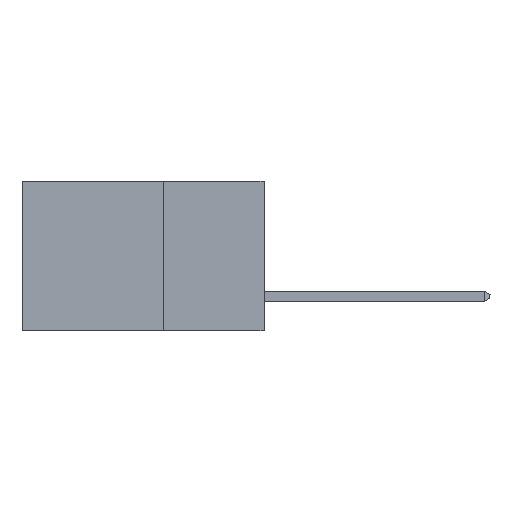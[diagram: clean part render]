
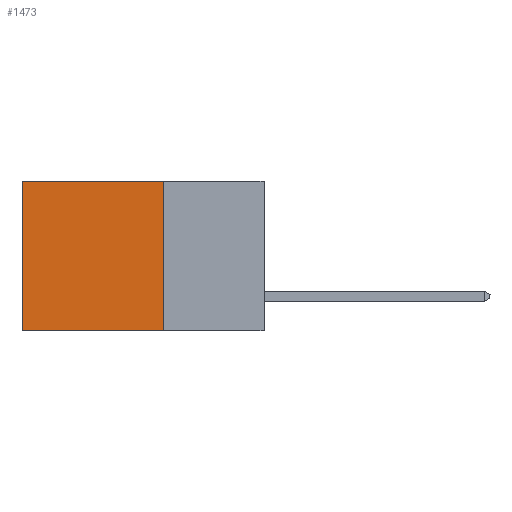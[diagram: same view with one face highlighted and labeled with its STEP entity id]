
A CAD part, left-side view. The second image highlights one B-rep face of the part: STEP entity #1473.
In plain terms, the highlighted planar face has unit normal (-1, 0, 0).
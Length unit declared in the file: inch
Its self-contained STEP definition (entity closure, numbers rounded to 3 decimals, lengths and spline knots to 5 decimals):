
#175 = CARTESIAN_POINT ( 'NONE',  ( 0.2615, 0.25, -0.37 ) ) ;
#930 = VECTOR ( 'NONE', #11636, 39.37008 ) ;
#1304 = EDGE_LOOP ( 'NONE', ( #3602, #11154, #7606, #9741 ) ) ;
#1473 = ADVANCED_FACE ( 'NONE', ( #2576 ), #13557, .F. ) ;
#1563 = DIRECTION ( 'NONE',  ( 0., 0., -1. ) ) ;
#2576 = FACE_OUTER_BOUND ( 'NONE', #1304, .T. ) ;
#3214 = CARTESIAN_POINT ( 'NONE',  ( 0.2615, 0.25, -0.37 ) ) ;
#3551 = CARTESIAN_POINT ( 'NONE',  ( 0.2615, 0.25, 0. ) ) ;
#3602 = ORIENTED_EDGE ( 'NONE', *, *, #7411, .T. ) ;
#3848 = LINE ( 'NONE', #4694, #7327 ) ;
#3891 = CARTESIAN_POINT ( 'NONE',  ( 0.2615, 0.6, -0.37 ) ) ;
#3955 = LINE ( 'NONE', #5013, #13419 ) ;
#4158 = DIRECTION ( 'NONE',  ( 1., 0., 0. ) ) ;
#4160 = EDGE_CURVE ( 'NONE', #10025, #10816, #3955, .T. ) ;
#4694 = CARTESIAN_POINT ( 'NONE',  ( 0.2615, 0.6, -0.37 ) ) ;
#5013 = CARTESIAN_POINT ( 'NONE',  ( 0.2615, 0.25, -0.37 ) ) ;
#5068 = VERTEX_POINT ( 'NONE', #3891 ) ;
#5295 = LINE ( 'NONE', #13931, #12448 ) ;
#6496 = DIRECTION ( 'NONE',  ( 0., 1., 0. ) ) ;
#7198 = AXIS2_PLACEMENT_3D ( 'NONE', #175, #4158, #10491 ) ;
#7296 = LINE ( 'NONE', #12596, #930 ) ;
#7327 = VECTOR ( 'NONE', #8037, 39.37008 ) ;
#7411 = EDGE_CURVE ( 'NONE', #12494, #5068, #3848, .T. ) ;
#7606 = ORIENTED_EDGE ( 'NONE', *, *, #4160, .F. ) ;
#7935 = EDGE_CURVE ( 'NONE', #10025, #12494, #7296, .T. ) ;
#8037 = DIRECTION ( 'NONE',  ( 0., 0., -1. ) ) ;
#9741 = ORIENTED_EDGE ( 'NONE', *, *, #7935, .T. ) ;
#10025 = VERTEX_POINT ( 'NONE', #3551 ) ;
#10491 = DIRECTION ( 'NONE',  ( 0., 0., -1. ) ) ;
#10816 = VERTEX_POINT ( 'NONE', #3214 ) ;
#11154 = ORIENTED_EDGE ( 'NONE', *, *, #13673, .F. ) ;
#11636 = DIRECTION ( 'NONE',  ( 0., 1., 0. ) ) ;
#12144 = CARTESIAN_POINT ( 'NONE',  ( 0.2615, 0.6, 0. ) ) ;
#12448 = VECTOR ( 'NONE', #6496, 39.37008 ) ;
#12494 = VERTEX_POINT ( 'NONE', #12144 ) ;
#12596 = CARTESIAN_POINT ( 'NONE',  ( 0.2615, 0.25, 0. ) ) ;
#13419 = VECTOR ( 'NONE', #1563, 39.37008 ) ;
#13557 = PLANE ( 'NONE',  #7198 ) ;
#13673 = EDGE_CURVE ( 'NONE', #10816, #5068, #5295, .T. ) ;
#13931 = CARTESIAN_POINT ( 'NONE',  ( 0.2615, 0.25, -0.37 ) ) ;
